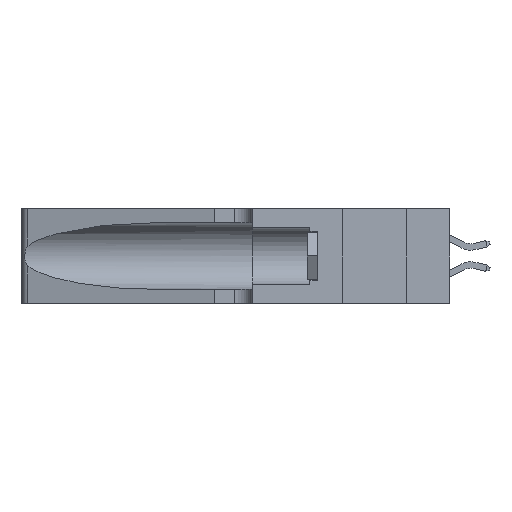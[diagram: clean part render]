
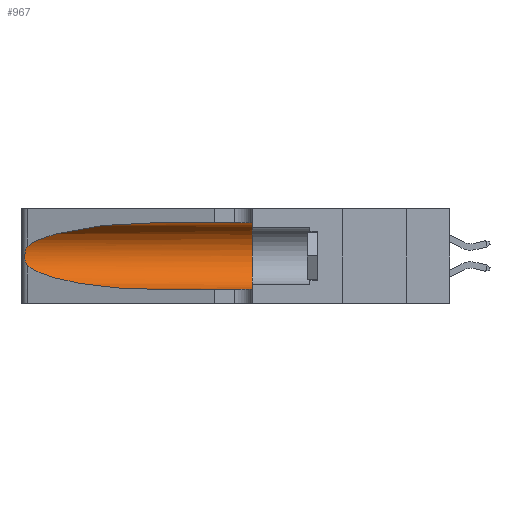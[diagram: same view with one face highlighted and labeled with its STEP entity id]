
A CAD part, left-side view. The second image highlights one B-rep face of the part: STEP entity #967.
In plain terms, the highlighted cylindrical face has radius 3.308 mm (diameter 6.617 mm), a partial arc.
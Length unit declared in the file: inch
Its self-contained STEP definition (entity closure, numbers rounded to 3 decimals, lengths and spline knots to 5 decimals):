
#551 = ORIENTED_EDGE ( 'NONE', *, *, #19543, .T. ) ;
#946 = CARTESIAN_POINT ( 'NONE',  ( 0.25487, 1.22718, 0.22369 ) ) ;
#967 = ADVANCED_FACE ( 'NONE', ( #15557 ), #12608, .F. ) ;
#3244 = CARTESIAN_POINT ( 'NONE',  ( 0.25487, 1.22718, 0.22369 ) ) ;
#3932 = CARTESIAN_POINT ( 'NONE',  ( 0.18966, 0.96281, 0.31525 ) ) ;
#4069 = ORIENTED_EDGE ( 'NONE', *, *, #39312, .F. ) ;
#5391 = CARTESIAN_POINT ( 'NONE',  ( 0.25639, 1.23186, 0.15144 ) ) ;
#5418 = VERTEX_POINT ( 'NONE', #32374 ) ;
#5674 = CARTESIAN_POINT ( 'NONE',  ( 0.1305, 0.72297, 0.31525 ) ) ;
#6584 = CARTESIAN_POINT ( 'NONE',  ( 0.1305, 0.72297, 0.05475 ) ) ;
#7993 = CIRCLE ( 'NONE', #11979, 0.13025 ) ;
#8208 = DIRECTION ( 'NONE',  ( 0., -1., 0. ) ) ;
#8465 = CARTESIAN_POINT ( 'NONE',  ( 0.25555, 1.22993, 0.14849 ) ) ;
#8702 =( BOUNDED_CURVE ( )  B_SPLINE_CURVE ( 3, ( #16521, #39785, #27635, #28396 ),
 .UNSPECIFIED., .F., .F. ) 
 B_SPLINE_CURVE_WITH_KNOTS ( ( 4, 4 ),
 ( 3.44316, 4.71239 ),
 .UNSPECIFIED. ) 
 CURVE ( )  GEOMETRIC_REPRESENTATION_ITEM ( )  RATIONAL_B_SPLINE_CURVE ( ( 1., 0.87, 0.87, 1. ) ) 
 REPRESENTATION_ITEM ( '' )  );
#8800 = CARTESIAN_POINT ( 'NONE',  ( 0.1305, 1.61858, 0.31525 ) ) ;
#9333 = CARTESIAN_POINT ( 'NONE',  ( 0.1305, 1.61858, 0.185 ) ) ;
#10466 =( BOUNDED_CURVE ( )  B_SPLINE_CURVE ( 3, ( #22486, #3932, #25583, #946 ),
 .UNSPECIFIED., .F., .F. ) 
 B_SPLINE_CURVE_WITH_KNOTS ( ( 4, 4 ),
 ( 1.5708, 2.84003 ),
 .UNSPECIFIED. ) 
 CURVE ( )  GEOMETRIC_REPRESENTATION_ITEM ( )  RATIONAL_B_SPLINE_CURVE ( ( 1., 0.87, 0.87, 1. ) ) 
 REPRESENTATION_ITEM ( '' )  );
#11838 = CARTESIAN_POINT ( 'NONE',  ( 0.1305, 1.61858, 0.05475 ) ) ;
#11979 = AXIS2_PLACEMENT_3D ( 'NONE', #26176, #23323, #13525 ) ;
#12608 = CYLINDRICAL_SURFACE ( 'NONE', #14267, 0.13025 ) ;
#12774 = EDGE_LOOP ( 'NONE', ( #551, #37200, #39543, #26311, #39235, #4069 ) ) ;
#13042 = CARTESIAN_POINT ( 'NONE',  ( 0.25787, 1.23484, 0.2124 ) ) ;
#13525 = DIRECTION ( 'NONE',  ( 0., 0., 1. ) ) ;
#13702 = VERTEX_POINT ( 'NONE', #31696 ) ;
#14267 = AXIS2_PLACEMENT_3D ( 'NONE', #9333, #37307, #36787 ) ;
#14982 = VERTEX_POINT ( 'NONE', #38106 ) ;
#15557 = FACE_OUTER_BOUND ( 'NONE', #12774, .T. ) ;
#16304 = CARTESIAN_POINT ( 'NONE',  ( 0.26018, 1.23835, 0.19895 ) ) ;
#16521 = CARTESIAN_POINT ( 'NONE',  ( 0.25487, 1.22718, 0.14631 ) ) ;
#18790 = VECTOR ( 'NONE', #8208, 39.37008 ) ;
#19543 = EDGE_CURVE ( 'NONE', #30119, #13702, #10466, .T. ) ;
#20944 = CARTESIAN_POINT ( 'NONE',  ( 0.25487, 1.22718, 0.14631 ) ) ;
#22486 = CARTESIAN_POINT ( 'NONE',  ( 0.1305, 0.72297, 0.31525 ) ) ;
#23323 = DIRECTION ( 'NONE',  ( 0., 1., 0. ) ) ;
#23374 = EDGE_CURVE ( 'NONE', #14982, #30241, #8702, .T. ) ;
#25034 = VERTEX_POINT ( 'NONE', #30710 ) ;
#25388 = CARTESIAN_POINT ( 'NONE',  ( 0.25555, 1.22994, 0.2215 ) ) ;
#25583 = CARTESIAN_POINT ( 'NONE',  ( 0.2373, 1.15595, 0.28018 ) ) ;
#26176 = CARTESIAN_POINT ( 'NONE',  ( 0.1305, 0.35, 0.185 ) ) ;
#26311 = ORIENTED_EDGE ( 'NONE', *, *, #35020, .T. ) ;
#27049 = LINE ( 'NONE', #11838, #18790 ) ;
#27635 = CARTESIAN_POINT ( 'NONE',  ( 0.18966, 0.96281, 0.05475 ) ) ;
#28396 = CARTESIAN_POINT ( 'NONE',  ( 0.1305, 0.72297, 0.05475 ) ) ;
#28502 = CARTESIAN_POINT ( 'NONE',  ( 0.25639, 1.23184, 0.21858 ) ) ;
#29845 = CARTESIAN_POINT ( 'NONE',  ( 0.25789, 1.23486, 0.15765 ) ) ;
#29848 = VECTOR ( 'NONE', #36923, 39.37008 ) ;
#29969 = CARTESIAN_POINT ( 'NONE',  ( 0.25856, 1.23593, 0.16098 ) ) ;
#30086 = EDGE_CURVE ( 'NONE', #13702, #14982, #33744, .T. ) ;
#30119 = VERTEX_POINT ( 'NONE', #5674 ) ;
#30241 = VERTEX_POINT ( 'NONE', #6584 ) ;
#30710 = CARTESIAN_POINT ( 'NONE',  ( 0.1305, 0.35, 0.31525 ) ) ;
#31696 = CARTESIAN_POINT ( 'NONE',  ( 0.25487, 1.22718, 0.22369 ) ) ;
#31716 = CARTESIAN_POINT ( 'NONE',  ( 0.25854, 1.2359, 0.20912 ) ) ;
#32269 = CARTESIAN_POINT ( 'NONE',  ( 0.26075, 1.23896, 0.178 ) ) ;
#32374 = CARTESIAN_POINT ( 'NONE',  ( 0.1305, 0.35, 0.05475 ) ) ;
#33744 = B_SPLINE_CURVE_WITH_KNOTS ( 'NONE', 3,
 ( #3244, #25388, #28502, #13042, #31716, #16304, #34925, #32269, #35915, #29969, #29845, #5391, #8465, #20944 ),
 .UNSPECIFIED., .F., .F.,
 ( 4, 2, 2, 2, 2, 2, 4 ),
 ( 0., 0.00027, 0.00053, 0.00107, 0.0016, 0.00187, 0.00214 ),
 .UNSPECIFIED. ) ;
#34925 = CARTESIAN_POINT ( 'NONE',  ( 0.26075, 1.23896, 0.19203 ) ) ;
#35020 = EDGE_CURVE ( 'NONE', #30241, #5418, #27049, .T. ) ;
#35915 = CARTESIAN_POINT ( 'NONE',  ( 0.26017, 1.23833, 0.17102 ) ) ;
#36483 = EDGE_CURVE ( 'NONE', #25034, #5418, #7993, .T. ) ;
#36787 = DIRECTION ( 'NONE',  ( 0., 0., -1. ) ) ;
#36923 = DIRECTION ( 'NONE',  ( 0., -1., 0. ) ) ;
#37200 = ORIENTED_EDGE ( 'NONE', *, *, #30086, .T. ) ;
#37307 = DIRECTION ( 'NONE',  ( 0., -1., 0. ) ) ;
#38071 = LINE ( 'NONE', #8800, #29848 ) ;
#38106 = CARTESIAN_POINT ( 'NONE',  ( 0.25487, 1.22718, 0.14631 ) ) ;
#39235 = ORIENTED_EDGE ( 'NONE', *, *, #36483, .F. ) ;
#39312 = EDGE_CURVE ( 'NONE', #30119, #25034, #38071, .T. ) ;
#39543 = ORIENTED_EDGE ( 'NONE', *, *, #23374, .T. ) ;
#39785 = CARTESIAN_POINT ( 'NONE',  ( 0.2373, 1.15595, 0.08982 ) ) ;
